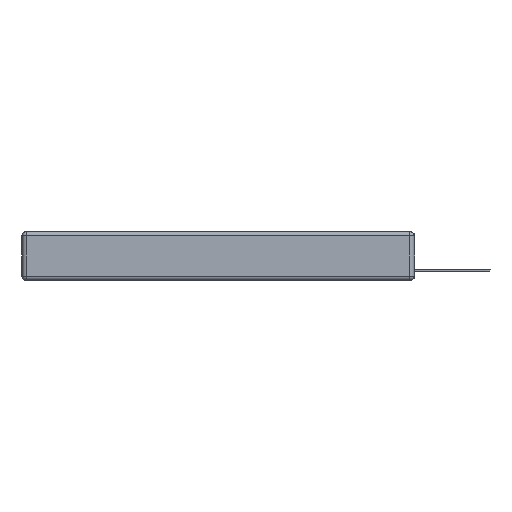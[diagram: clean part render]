
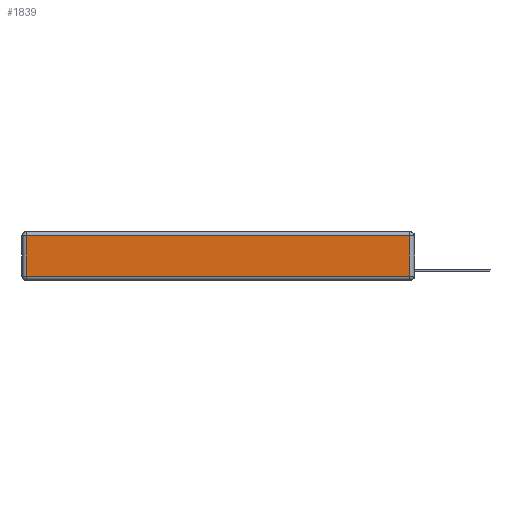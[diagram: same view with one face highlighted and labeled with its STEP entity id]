
A CAD part, left-side view. The second image highlights one B-rep face of the part: STEP entity #1839.
In plain terms, the highlighted planar face has unit normal (-1, 0, 0).
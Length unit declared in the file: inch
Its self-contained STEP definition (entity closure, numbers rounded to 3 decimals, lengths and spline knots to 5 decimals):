
#546 = EDGE_CURVE ( 'NONE', #1501, #1573, #3706, .T. ) ;
#693 = DIRECTION ( 'NONE',  ( 0., 0., 1. ) ) ;
#1244 = VECTOR ( 'NONE', #5527, 39.37008 ) ;
#1288 = CARTESIAN_POINT ( 'NONE',  ( 0., 0.03, -0.343 ) ) ;
#1432 = VERTEX_POINT ( 'NONE', #7010 ) ;
#1501 = VERTEX_POINT ( 'NONE', #10235 ) ;
#1573 = VERTEX_POINT ( 'NONE', #15044 ) ;
#1839 = ADVANCED_FACE ( 'NONE', ( #6811 ), #3866, .T. ) ;
#3706 = LINE ( 'NONE', #10427, #1244 ) ;
#3866 = PLANE ( 'NONE',  #16143 ) ;
#4327 = DIRECTION ( 'NONE',  ( 0., -1., 0. ) ) ;
#4508 = DIRECTION ( 'NONE',  ( 0., 0., 1. ) ) ;
#5248 = LINE ( 'NONE', #13282, #6718 ) ;
#5442 = ORIENTED_EDGE ( 'NONE', *, *, #13373, .T. ) ;
#5527 = DIRECTION ( 'NONE',  ( 0., 1., 0. ) ) ;
#6560 = LINE ( 'NONE', #13612, #18369 ) ;
#6718 = VECTOR ( 'NONE', #13143, 39.37008 ) ;
#6811 = FACE_OUTER_BOUND ( 'NONE', #18854, .T. ) ;
#7010 = CARTESIAN_POINT ( 'NONE',  ( 0., 2.72, -0.313 ) ) ;
#8170 = ORIENTED_EDGE ( 'NONE', *, *, #546, .T. ) ;
#9022 = ORIENTED_EDGE ( 'NONE', *, *, #10738, .T. ) ;
#10097 = DIRECTION ( 'NONE',  ( -1., 0., 0. ) ) ;
#10235 = CARTESIAN_POINT ( 'NONE',  ( 0., 0.03, -0.03 ) ) ;
#10427 = CARTESIAN_POINT ( 'NONE',  ( 0., 2.75, -0.03 ) ) ;
#10738 = EDGE_CURVE ( 'NONE', #1573, #1432, #5248, .T. ) ;
#12673 = EDGE_CURVE ( 'NONE', #1432, #17310, #6560, .T. ) ;
#13143 = DIRECTION ( 'NONE',  ( 0., 0., -1. ) ) ;
#13282 = CARTESIAN_POINT ( 'NONE',  ( 0., 2.72, -0.343 ) ) ;
#13373 = EDGE_CURVE ( 'NONE', #17310, #1501, #19077, .T. ) ;
#13612 = CARTESIAN_POINT ( 'NONE',  ( 0., 0., -0.313 ) ) ;
#15044 = CARTESIAN_POINT ( 'NONE',  ( 0., 2.72, -0.03 ) ) ;
#16143 = AXIS2_PLACEMENT_3D ( 'NONE', #16347, #10097, #693 ) ;
#16347 = CARTESIAN_POINT ( 'NONE',  ( 0., 0., -0.343 ) ) ;
#17038 = ORIENTED_EDGE ( 'NONE', *, *, #12673, .T. ) ;
#17310 = VERTEX_POINT ( 'NONE', #19147 ) ;
#17349 = VECTOR ( 'NONE', #4508, 39.37008 ) ;
#18369 = VECTOR ( 'NONE', #4327, 39.37008 ) ;
#18854 = EDGE_LOOP ( 'NONE', ( #17038, #5442, #8170, #9022 ) ) ;
#19077 = LINE ( 'NONE', #1288, #17349 ) ;
#19147 = CARTESIAN_POINT ( 'NONE',  ( 0., 0.03, -0.313 ) ) ;
